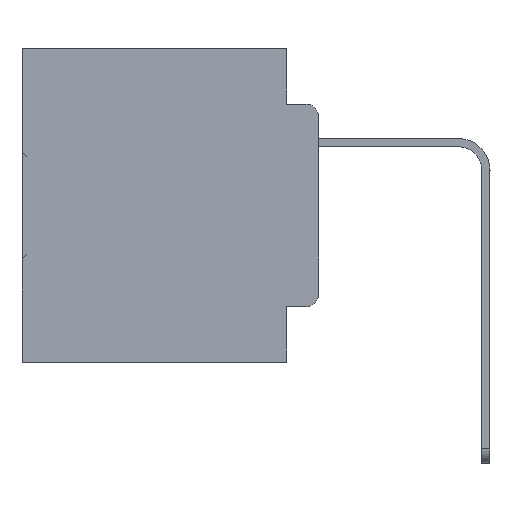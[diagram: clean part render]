
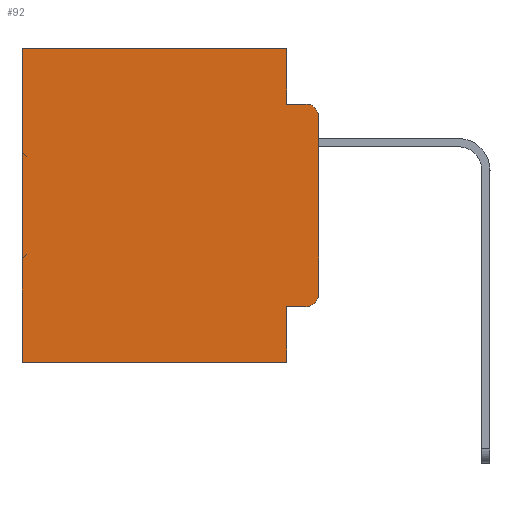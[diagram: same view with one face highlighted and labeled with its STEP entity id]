
A CAD part, left-side view. The second image highlights one B-rep face of the part: STEP entity #92.
In plain terms, the highlighted planar face has unit normal (-1, 0, 0).
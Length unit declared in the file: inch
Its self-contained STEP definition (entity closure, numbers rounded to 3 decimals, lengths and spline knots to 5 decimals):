
#92 = ADVANCED_FACE ( 'NONE', ( #9297 ), #30810, .F. ) ;
#265 = DIRECTION ( 'NONE',  ( 1., 0., 0. ) ) ;
#382 = EDGE_CURVE ( 'NONE', #5775, #30842, #10569, .T. ) ;
#584 = VERTEX_POINT ( 'NONE', #35479 ) ;
#795 = LINE ( 'NONE', #1132, #21951 ) ;
#840 = DIRECTION ( 'NONE',  ( -1., 0., 0. ) ) ;
#1132 = CARTESIAN_POINT ( 'NONE',  ( 0.298, 0., -0.5 ) ) ;
#1358 = LINE ( 'NONE', #29379, #23799 ) ;
#1525 = CARTESIAN_POINT ( 'NONE',  ( 0.298, 0.051, 0. ) ) ;
#1557 = EDGE_CURVE ( 'NONE', #12973, #3631, #26116, .T. ) ;
#1579 = CARTESIAN_POINT ( 'NONE',  ( 0.298, 0.051, 0. ) ) ;
#1707 = VERTEX_POINT ( 'NONE', #22981 ) ;
#1847 = VERTEX_POINT ( 'NONE', #20654 ) ;
#2245 = EDGE_CURVE ( 'NONE', #30770, #1847, #10058, .T. ) ;
#3631 = VERTEX_POINT ( 'NONE', #27157 ) ;
#4055 = EDGE_LOOP ( 'NONE', ( #16850, #20072, #19225, #12271, #5951, #6101, #20188, #5401, #4150, #7630 ) ) ;
#4150 = ORIENTED_EDGE ( 'NONE', *, *, #23365, .T. ) ;
#4628 = VERTEX_POINT ( 'NONE', #21588 ) ;
#4644 = AXIS2_PLACEMENT_3D ( 'NONE', #19782, #33466, #11839 ) ;
#4663 = DIRECTION ( 'NONE',  ( 0., 1., 0. ) ) ;
#4866 = DIRECTION ( 'NONE',  ( 0., -1., 0. ) ) ;
#5401 = ORIENTED_EDGE ( 'NONE', *, *, #6969, .F. ) ;
#5537 = LINE ( 'NONE', #27897, #34915 ) ;
#5700 = CARTESIAN_POINT ( 'NONE',  ( 0.298, 0.051, 0. ) ) ;
#5775 = VERTEX_POINT ( 'NONE', #5700 ) ;
#5907 = CIRCLE ( 'NONE', #25959, 0.02 ) ;
#5951 = ORIENTED_EDGE ( 'NONE', *, *, #13394, .T. ) ;
#6101 = ORIENTED_EDGE ( 'NONE', *, *, #1557, .T. ) ;
#6416 = VECTOR ( 'NONE', #31340, 39.37008 ) ;
#6969 = EDGE_CURVE ( 'NONE', #1707, #4628, #18452, .T. ) ;
#7475 = VECTOR ( 'NONE', #4866, 39.37008 ) ;
#7630 = ORIENTED_EDGE ( 'NONE', *, *, #2245, .T. ) ;
#8491 = CARTESIAN_POINT ( 'NONE',  ( 0.298, 0., 0. ) ) ;
#9297 = FACE_OUTER_BOUND ( 'NONE', #4055, .T. ) ;
#10058 = CIRCLE ( 'NONE', #4644, 0.02 ) ;
#10569 = LINE ( 'NONE', #1579, #26554 ) ;
#10998 = DIRECTION ( 'NONE',  ( 0., 0., -1. ) ) ;
#11355 = DIRECTION ( 'NONE',  ( 0., 0., -1. ) ) ;
#11839 = DIRECTION ( 'NONE',  ( 0., 0., -1. ) ) ;
#12271 = ORIENTED_EDGE ( 'NONE', *, *, #382, .F. ) ;
#12842 = VECTOR ( 'NONE', #13556, 39.37008 ) ;
#12973 = VERTEX_POINT ( 'NONE', #24114 ) ;
#13394 = EDGE_CURVE ( 'NONE', #5775, #12973, #1358, .T. ) ;
#13556 = DIRECTION ( 'NONE',  ( 0., -1., 0. ) ) ;
#14598 = CARTESIAN_POINT ( 'NONE',  ( 0.298, 0.02, -0.1085 ) ) ;
#16850 = ORIENTED_EDGE ( 'NONE', *, *, #21379, .F. ) ;
#16856 = CARTESIAN_POINT ( 'NONE',  ( 0.298, 0.473, 0. ) ) ;
#18452 = LINE ( 'NONE', #1525, #6416 ) ;
#18474 = CARTESIAN_POINT ( 'NONE',  ( 0.298, 0.051, -0.0885 ) ) ;
#18857 = EDGE_CURVE ( 'NONE', #30842, #584, #29462, .T. ) ;
#18950 = CARTESIAN_POINT ( 'NONE',  ( 0.298, 0.051, -0.4115 ) ) ;
#19225 = ORIENTED_EDGE ( 'NONE', *, *, #18857, .F. ) ;
#19612 = CARTESIAN_POINT ( 'NONE',  ( 0.298, 0.02, -0.4115 ) ) ;
#19658 = CARTESIAN_POINT ( 'NONE',  ( 0.298, 0., -0.1085 ) ) ;
#19782 = CARTESIAN_POINT ( 'NONE',  ( 0.298, 0.02, -0.3915 ) ) ;
#20072 = ORIENTED_EDGE ( 'NONE', *, *, #24090, .T. ) ;
#20188 = ORIENTED_EDGE ( 'NONE', *, *, #20825, .F. ) ;
#20654 = CARTESIAN_POINT ( 'NONE',  ( 0.298, 0., -0.3915 ) ) ;
#20825 = EDGE_CURVE ( 'NONE', #4628, #3631, #795, .T. ) ;
#21379 = EDGE_CURVE ( 'NONE', #32733, #1847, #5537, .T. ) ;
#21588 = CARTESIAN_POINT ( 'NONE',  ( 0.298, 0.051, -0.5 ) ) ;
#21951 = VECTOR ( 'NONE', #23324, 39.37008 ) ;
#22981 = CARTESIAN_POINT ( 'NONE',  ( 0.298, 0.051, -0.4115 ) ) ;
#23324 = DIRECTION ( 'NONE',  ( 0., 1., 0. ) ) ;
#23365 = EDGE_CURVE ( 'NONE', #1707, #30770, #35315, .T. ) ;
#23799 = VECTOR ( 'NONE', #4663, 39.37008 ) ;
#24090 = EDGE_CURVE ( 'NONE', #32733, #584, #5907, .T. ) ;
#24114 = CARTESIAN_POINT ( 'NONE',  ( 0.298, 0.473, 0. ) ) ;
#25526 = DIRECTION ( 'NONE',  ( 0., 0., -1. ) ) ;
#25959 = AXIS2_PLACEMENT_3D ( 'NONE', #14598, #840, #28338 ) ;
#26116 = LINE ( 'NONE', #16856, #26973 ) ;
#26441 = DIRECTION ( 'NONE',  ( 0., 0., -1. ) ) ;
#26554 = VECTOR ( 'NONE', #26441, 39.37008 ) ;
#26973 = VECTOR ( 'NONE', #25526, 39.37008 ) ;
#27157 = CARTESIAN_POINT ( 'NONE',  ( 0.298, 0.473, -0.5 ) ) ;
#27897 = CARTESIAN_POINT ( 'NONE',  ( 0.298, 0., 0. ) ) ;
#28338 = DIRECTION ( 'NONE',  ( 0., 0., -1. ) ) ;
#29379 = CARTESIAN_POINT ( 'NONE',  ( 0.298, 0., 0. ) ) ;
#29462 = LINE ( 'NONE', #18474, #7475 ) ;
#30508 = CARTESIAN_POINT ( 'NONE',  ( 0.298, 0.051, -0.0885 ) ) ;
#30770 = VERTEX_POINT ( 'NONE', #19612 ) ;
#30810 = PLANE ( 'NONE',  #32166 ) ;
#30842 = VERTEX_POINT ( 'NONE', #30508 ) ;
#31340 = DIRECTION ( 'NONE',  ( 0., 0., -1. ) ) ;
#32166 = AXIS2_PLACEMENT_3D ( 'NONE', #8491, #265, #11355 ) ;
#32733 = VERTEX_POINT ( 'NONE', #19658 ) ;
#33466 = DIRECTION ( 'NONE',  ( -1., 0., 0. ) ) ;
#34915 = VECTOR ( 'NONE', #10998, 39.37008 ) ;
#35315 = LINE ( 'NONE', #18950, #12842 ) ;
#35479 = CARTESIAN_POINT ( 'NONE',  ( 0.298, 0.02, -0.0885 ) ) ;
